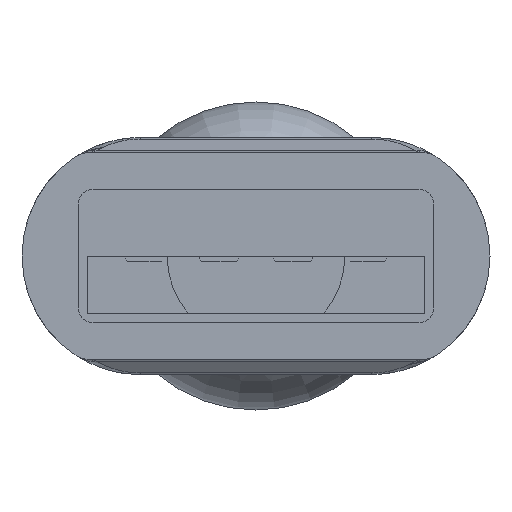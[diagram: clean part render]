
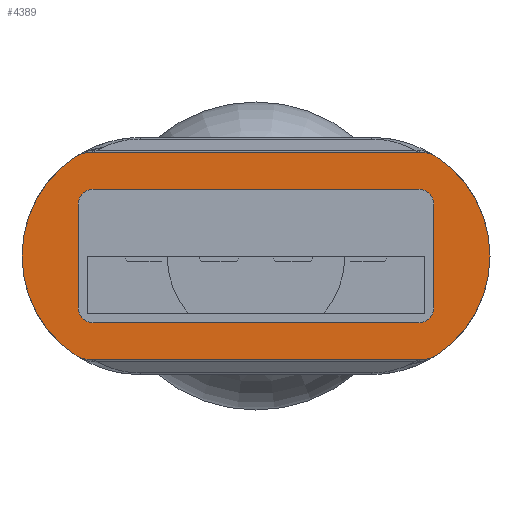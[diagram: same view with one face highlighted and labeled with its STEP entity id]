
A CAD part, left-side view. The second image highlights one B-rep face of the part: STEP entity #4389.
In plain terms, the highlighted planar face has unit normal (-1, 0, 0).
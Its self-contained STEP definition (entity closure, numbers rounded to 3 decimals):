
#5 = CIRCLE ( 'NONE', #3071, 0.5 ) ;
#41 = CARTESIAN_POINT ( 'NONE',  ( -67., -5.558, -3.5 ) ) ;
#51 = VERTEX_POINT ( 'NONE', #3926 ) ;
#92 = CIRCLE ( 'NONE', #192, 0.5 ) ;
#119 = AXIS2_PLACEMENT_3D ( 'NONE', #4304, #1485, #4464 ) ;
#156 = CIRCLE ( 'NONE', #4570, 1. ) ;
#165 = LINE ( 'NONE', #2789, #5486 ) ;
#184 = VECTOR ( 'NONE', #2848, 1000. ) ;
#192 = AXIS2_PLACEMENT_3D ( 'NONE', #545, #3593, #4831 ) ;
#209 = EDGE_CURVE ( 'NONE', #1467, #2275, #4296, .T. ) ;
#231 = CARTESIAN_POINT ( 'NONE',  ( -67., 5.5, -2.25 ) ) ;
#236 = CIRCLE ( 'NONE', #960, 1. ) ;
#241 = ORIENTED_EDGE ( 'NONE', *, *, #2312, .T. ) ;
#285 = DIRECTION ( 'NONE',  ( 0., 0., -1. ) ) ;
#337 = EDGE_CURVE ( 'NONE', #5076, #1569, #953, .T. ) ;
#389 = CARTESIAN_POINT ( 'NONE',  ( -67., -3.9, 0. ) ) ;
#445 = DIRECTION ( 'NONE',  ( 0., 1., 0. ) ) ;
#469 = VERTEX_POINT ( 'NONE', #2366 ) ;
#480 = CARTESIAN_POINT ( 'NONE',  ( -67., 6., 1.75 ) ) ;
#516 = DIRECTION ( 'NONE',  ( 1., 0., 0. ) ) ;
#543 = CARTESIAN_POINT ( 'NONE',  ( -67., 5.558, 2.5 ) ) ;
#545 = CARTESIAN_POINT ( 'NONE',  ( -67., -5.5, -1.75 ) ) ;
#578 = ORIENTED_EDGE ( 'NONE', *, *, #5351, .T. ) ;
#660 = VECTOR ( 'NONE', #1307, 1000. ) ;
#731 = EDGE_CURVE ( 'NONE', #4526, #1467, #1414, .T. ) ;
#838 = CIRCLE ( 'NONE', #5432, 0.5 ) ;
#902 = VERTEX_POINT ( 'NONE', #2498 ) ;
#953 = LINE ( 'NONE', #4395, #2586 ) ;
#960 = AXIS2_PLACEMENT_3D ( 'NONE', #4401, #1873, #1077 ) ;
#985 = AXIS2_PLACEMENT_3D ( 'NONE', #1199, #4580, #3762 ) ;
#1033 = DIRECTION ( 'NONE',  ( -1., 0., 0. ) ) ;
#1038 = EDGE_CURVE ( 'NONE', #1769, #4526, #236, .T. ) ;
#1077 = DIRECTION ( 'NONE',  ( 0., 1., 0. ) ) ;
#1088 = CARTESIAN_POINT ( 'NONE',  ( -67., 6., -2.25 ) ) ;
#1102 = CARTESIAN_POINT ( 'NONE',  ( -67., 5.5, 2.25 ) ) ;
#1105 = CARTESIAN_POINT ( 'NONE',  ( -67., 5.558, -2.5 ) ) ;
#1195 = EDGE_CURVE ( 'NONE', #4633, #1576, #2877, .T. ) ;
#1199 = CARTESIAN_POINT ( 'NONE',  ( -67., -5.558, 2.5 ) ) ;
#1258 = VECTOR ( 'NONE', #1852, 1000. ) ;
#1307 = DIRECTION ( 'NONE',  ( 0., -1., 0. ) ) ;
#1308 = VERTEX_POINT ( 'NONE', #4620 ) ;
#1339 = CARTESIAN_POINT ( 'NONE',  ( -67., -6., -2.25 ) ) ;
#1386 = DIRECTION ( 'NONE',  ( 0., 1., 0. ) ) ;
#1414 = CIRCLE ( 'NONE', #2130, 4. ) ;
#1461 = CARTESIAN_POINT ( 'NONE',  ( -67., -6.111, -3.333 ) ) ;
#1467 = VERTEX_POINT ( 'NONE', #2760 ) ;
#1485 = DIRECTION ( 'NONE',  ( -1., 0., 0. ) ) ;
#1548 = CARTESIAN_POINT ( 'NONE',  ( -67., -5.5, -2.25 ) ) ;
#1557 = EDGE_CURVE ( 'NONE', #1769, #1308, #165, .T. ) ;
#1569 = VERTEX_POINT ( 'NONE', #2682 ) ;
#1576 = VERTEX_POINT ( 'NONE', #1102 ) ;
#1745 = PLANE ( 'NONE',  #119 ) ;
#1769 = VERTEX_POINT ( 'NONE', #41 ) ;
#1777 = CARTESIAN_POINT ( 'NONE',  ( -67., -3.9, 0. ) ) ;
#1826 = CARTESIAN_POINT ( 'NONE',  ( -67., 5.5, -1.75 ) ) ;
#1852 = DIRECTION ( 'NONE',  ( 0., 0., 1. ) ) ;
#1859 = EDGE_LOOP ( 'NONE', ( #3823, #5031, #3872, #4717, #4441, #4784, #578, #2156, #4210 ) ) ;
#1873 = DIRECTION ( 'NONE',  ( -1., 0., 0. ) ) ;
#2024 = DIRECTION ( 'NONE',  ( 0., -1., 0. ) ) ;
#2083 = CARTESIAN_POINT ( 'NONE',  ( -67., -5.5, 1.75 ) ) ;
#2101 = ORIENTED_EDGE ( 'NONE', *, *, #2771, .T. ) ;
#2130 = AXIS2_PLACEMENT_3D ( 'NONE', #1777, #1033, #4864 ) ;
#2156 = ORIENTED_EDGE ( 'NONE', *, *, #1557, .F. ) ;
#2207 = CARTESIAN_POINT ( 'NONE',  ( -67., 3.9, 0. ) ) ;
#2244 = DIRECTION ( 'NONE',  ( 0., 1., 0. ) ) ;
#2250 = EDGE_CURVE ( 'NONE', #469, #2994, #92, .T. ) ;
#2271 = DIRECTION ( 'NONE',  ( 0., 1., 0. ) ) ;
#2275 = VERTEX_POINT ( 'NONE', #3932 ) ;
#2294 = EDGE_CURVE ( 'NONE', #2702, #1576, #5, .T. ) ;
#2312 = EDGE_CURVE ( 'NONE', #2459, #51, #3789, .T. ) ;
#2326 = DIRECTION ( 'NONE',  ( 1., 0., 0. ) ) ;
#2366 = CARTESIAN_POINT ( 'NONE',  ( -67., -6., -1.75 ) ) ;
#2372 = CARTESIAN_POINT ( 'NONE',  ( -67., 6.111, -3.333 ) ) ;
#2398 = EDGE_CURVE ( 'NONE', #2702, #51, #4965, .T. ) ;
#2434 = CARTESIAN_POINT ( 'NONE',  ( -67., -5.5, 2.25 ) ) ;
#2459 = VERTEX_POINT ( 'NONE', #231 ) ;
#2475 = AXIS2_PLACEMENT_3D ( 'NONE', #543, #2773, #2271 ) ;
#2498 = CARTESIAN_POINT ( 'NONE',  ( -67., 6.111, 3.333 ) ) ;
#2506 = DIRECTION ( 'NONE',  ( 0., 1., 0. ) ) ;
#2515 = CIRCLE ( 'NONE', #985, 1. ) ;
#2548 = ORIENTED_EDGE ( 'NONE', *, *, #2294, .T. ) ;
#2563 = DIRECTION ( 'NONE',  ( -1., 0., 0. ) ) ;
#2569 = EDGE_CURVE ( 'NONE', #902, #3726, #3099, .T. ) ;
#2586 = VECTOR ( 'NONE', #2024, 1000. ) ;
#2682 = CARTESIAN_POINT ( 'NONE',  ( -67., -5.558, 3.5 ) ) ;
#2702 = VERTEX_POINT ( 'NONE', #480 ) ;
#2717 = DIRECTION ( 'NONE',  ( -1., 0., 0. ) ) ;
#2760 = CARTESIAN_POINT ( 'NONE',  ( -67., -7.9, 0. ) ) ;
#2771 = EDGE_CURVE ( 'NONE', #4633, #5296, #838, .T. ) ;
#2773 = DIRECTION ( 'NONE',  ( -1., 0., 0. ) ) ;
#2789 = CARTESIAN_POINT ( 'NONE',  ( -67., 0., -3.5 ) ) ;
#2848 = DIRECTION ( 'NONE',  ( 0., 1., 0. ) ) ;
#2877 = LINE ( 'NONE', #4144, #184 ) ;
#2891 = AXIS2_PLACEMENT_3D ( 'NONE', #1826, #516, #2244 ) ;
#2994 = VERTEX_POINT ( 'NONE', #1548 ) ;
#3003 = FACE_BOUND ( 'NONE', #4878, .T. ) ;
#3071 = AXIS2_PLACEMENT_3D ( 'NONE', #3957, #2326, #3147 ) ;
#3099 = CIRCLE ( 'NONE', #3905, 4. ) ;
#3147 = DIRECTION ( 'NONE',  ( 0., 1., 0. ) ) ;
#3195 = EDGE_CURVE ( 'NONE', #5076, #902, #5165, .T. ) ;
#3225 = LINE ( 'NONE', #4937, #1258 ) ;
#3328 = DIRECTION ( 'NONE',  ( -1., 0., 0. ) ) ;
#3356 = DIRECTION ( 'NONE',  ( 1., 0., 0. ) ) ;
#3398 = ORIENTED_EDGE ( 'NONE', *, *, #2398, .F. ) ;
#3473 = LINE ( 'NONE', #1339, #660 ) ;
#3474 = ORIENTED_EDGE ( 'NONE', *, *, #2250, .T. ) ;
#3593 = DIRECTION ( 'NONE',  ( 1., 0., 0. ) ) ;
#3726 = VERTEX_POINT ( 'NONE', #2372 ) ;
#3762 = DIRECTION ( 'NONE',  ( 0., 1., 0. ) ) ;
#3789 = CIRCLE ( 'NONE', #2891, 0.5 ) ;
#3823 = ORIENTED_EDGE ( 'NONE', *, *, #731, .T. ) ;
#3872 = ORIENTED_EDGE ( 'NONE', *, *, #4533, .T. ) ;
#3905 = AXIS2_PLACEMENT_3D ( 'NONE', #2207, #2717, #5214 ) ;
#3926 = CARTESIAN_POINT ( 'NONE',  ( -67., 6., -1.75 ) ) ;
#3932 = CARTESIAN_POINT ( 'NONE',  ( -67., -6.111, 3.333 ) ) ;
#3957 = CARTESIAN_POINT ( 'NONE',  ( -67., 5.5, 1.75 ) ) ;
#3961 = ORIENTED_EDGE ( 'NONE', *, *, #1195, .F. ) ;
#4144 = CARTESIAN_POINT ( 'NONE',  ( -67., -6., 2.25 ) ) ;
#4206 = AXIS2_PLACEMENT_3D ( 'NONE', #389, #2563, #445 ) ;
#4210 = ORIENTED_EDGE ( 'NONE', *, *, #1038, .T. ) ;
#4296 = CIRCLE ( 'NONE', #4206, 4. ) ;
#4304 = CARTESIAN_POINT ( 'NONE',  ( -67., 0., 0. ) ) ;
#4389 = ADVANCED_FACE ( 'NONE', ( #5138, #3003 ), #1745, .T. ) ;
#4395 = CARTESIAN_POINT ( 'NONE',  ( -67., 0., 3.5 ) ) ;
#4401 = CARTESIAN_POINT ( 'NONE',  ( -67., -5.558, -2.5 ) ) ;
#4441 = ORIENTED_EDGE ( 'NONE', *, *, #3195, .T. ) ;
#4464 = DIRECTION ( 'NONE',  ( 0., 1., 0. ) ) ;
#4483 = CARTESIAN_POINT ( 'NONE',  ( -67., -6., 1.75 ) ) ;
#4492 = EDGE_CURVE ( 'NONE', #469, #5296, #3225, .T. ) ;
#4512 = VECTOR ( 'NONE', #285, 1000. ) ;
#4523 = ORIENTED_EDGE ( 'NONE', *, *, #4492, .F. ) ;
#4526 = VERTEX_POINT ( 'NONE', #1461 ) ;
#4533 = EDGE_CURVE ( 'NONE', #2275, #1569, #2515, .T. ) ;
#4569 = DIRECTION ( 'NONE',  ( 0., 1., 0. ) ) ;
#4570 = AXIS2_PLACEMENT_3D ( 'NONE', #1105, #3328, #4569 ) ;
#4580 = DIRECTION ( 'NONE',  ( -1., 0., 0. ) ) ;
#4620 = CARTESIAN_POINT ( 'NONE',  ( -67., 5.558, -3.5 ) ) ;
#4633 = VERTEX_POINT ( 'NONE', #2434 ) ;
#4681 = CARTESIAN_POINT ( 'NONE',  ( -67., 5.558, 3.5 ) ) ;
#4708 = EDGE_CURVE ( 'NONE', #2459, #2994, #3473, .T. ) ;
#4717 = ORIENTED_EDGE ( 'NONE', *, *, #337, .F. ) ;
#4784 = ORIENTED_EDGE ( 'NONE', *, *, #2569, .T. ) ;
#4831 = DIRECTION ( 'NONE',  ( 0., 1., 0. ) ) ;
#4864 = DIRECTION ( 'NONE',  ( 0., 1., 0. ) ) ;
#4878 = EDGE_LOOP ( 'NONE', ( #3398, #2548, #3961, #2101, #4523, #3474, #5190, #241 ) ) ;
#4937 = CARTESIAN_POINT ( 'NONE',  ( -67., -6., -2.25 ) ) ;
#4965 = LINE ( 'NONE', #1088, #4512 ) ;
#5031 = ORIENTED_EDGE ( 'NONE', *, *, #209, .T. ) ;
#5076 = VERTEX_POINT ( 'NONE', #4681 ) ;
#5138 = FACE_OUTER_BOUND ( 'NONE', #1859, .T. ) ;
#5165 = CIRCLE ( 'NONE', #2475, 1. ) ;
#5190 = ORIENTED_EDGE ( 'NONE', *, *, #4708, .F. ) ;
#5214 = DIRECTION ( 'NONE',  ( 0., 1., 0. ) ) ;
#5296 = VERTEX_POINT ( 'NONE', #4483 ) ;
#5351 = EDGE_CURVE ( 'NONE', #3726, #1308, #156, .T. ) ;
#5432 = AXIS2_PLACEMENT_3D ( 'NONE', #2083, #3356, #2506 ) ;
#5486 = VECTOR ( 'NONE', #1386, 1000. ) ;
